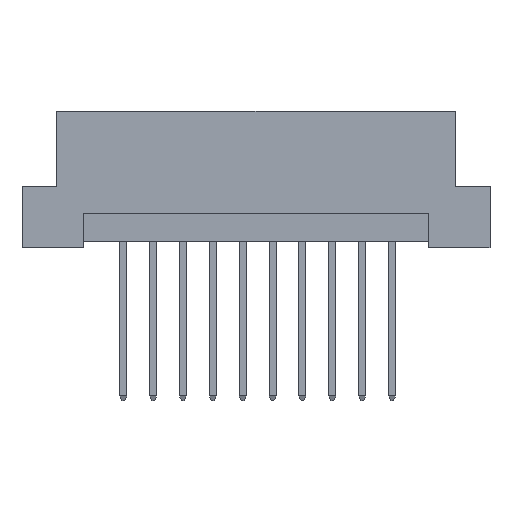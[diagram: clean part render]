
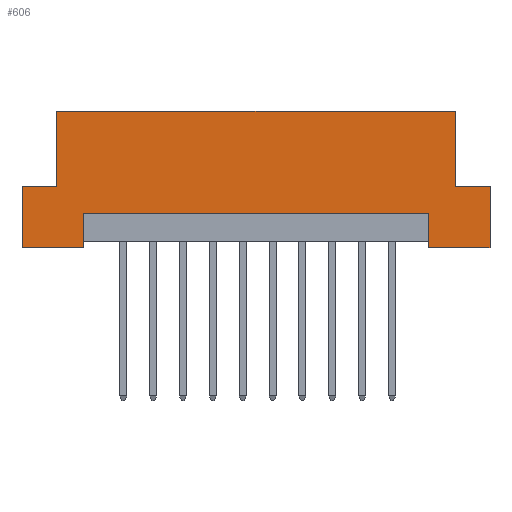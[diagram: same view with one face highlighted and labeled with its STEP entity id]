
A CAD part, front view. The second image highlights one B-rep face of the part: STEP entity #606.
In plain terms, the highlighted planar face has unit normal (0, -1, 0).
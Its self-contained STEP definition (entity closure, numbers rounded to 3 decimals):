
#6 = LINE ( 'NONE', #4077, #3075 ) ;
#26 = ORIENTED_EDGE ( 'NONE', *, *, #523, .F. ) ;
#90 = DIRECTION ( 'NONE',  ( -1., 0., 0. ) ) ;
#108 = DIRECTION ( 'NONE',  ( 0., 0., -1. ) ) ;
#235 = EDGE_CURVE ( 'NONE', #1384, #5717, #3863, .T. ) ;
#265 = VECTOR ( 'NONE', #2667, 1000. ) ;
#295 = CARTESIAN_POINT ( 'NONE',  ( -19.9, 0., 0. ) ) ;
#346 = EDGE_LOOP ( 'NONE', ( #26, #4946, #2214, #2042, #5143, #6350, #1174, #2642, #4425, #2897, #4144, #871 ) ) ;
#352 = LINE ( 'NONE', #419, #2236 ) ;
#419 = CARTESIAN_POINT ( 'NONE',  ( -19.9, 0., 0. ) ) ;
#425 = EDGE_CURVE ( 'NONE', #3949, #3758, #2984, .T. ) ;
#485 = DIRECTION ( 'NONE',  ( 0., 0., 1. ) ) ;
#523 = EDGE_CURVE ( 'NONE', #6024, #3803, #5255, .T. ) ;
#606 = ADVANCED_FACE ( 'NONE', ( #4904 ), #5379, .F. ) ;
#613 = LINE ( 'NONE', #5139, #684 ) ;
#618 = DIRECTION ( 'NONE',  ( 0., 0., -1. ) ) ;
#684 = VECTOR ( 'NONE', #108, 1000. ) ;
#708 = EDGE_CURVE ( 'NONE', #5141, #5516, #352, .T. ) ;
#871 = ORIENTED_EDGE ( 'NONE', *, *, #3981, .F. ) ;
#911 = DIRECTION ( 'NONE',  ( 1., 0., 0. ) ) ;
#1126 = CARTESIAN_POINT ( 'NONE',  ( 16.94, 0., 11.6 ) ) ;
#1157 = EDGE_CURVE ( 'NONE', #1899, #3949, #6, .T. ) ;
#1170 = VERTEX_POINT ( 'NONE', #6666 ) ;
#1174 = ORIENTED_EDGE ( 'NONE', *, *, #4488, .F. ) ;
#1384 = VERTEX_POINT ( 'NONE', #4988 ) ;
#1573 = CARTESIAN_POINT ( 'NONE',  ( -19.9, 0., 11.6 ) ) ;
#1659 = VECTOR ( 'NONE', #2355, 1000. ) ;
#1704 = CARTESIAN_POINT ( 'NONE',  ( -19.9, 0., 11.6 ) ) ;
#1819 = VECTOR ( 'NONE', #90, 1000. ) ;
#1820 = CARTESIAN_POINT ( 'NONE',  ( -14.69, 0., 0. ) ) ;
#1899 = VERTEX_POINT ( 'NONE', #6479 ) ;
#1977 = CARTESIAN_POINT ( 'NONE',  ( 19.9, 0., 0. ) ) ;
#2042 = ORIENTED_EDGE ( 'NONE', *, *, #425, .F. ) ;
#2144 = EDGE_CURVE ( 'NONE', #6024, #3431, #6234, .T. ) ;
#2214 = ORIENTED_EDGE ( 'NONE', *, *, #3253, .F. ) ;
#2236 = VECTOR ( 'NONE', #6577, 1000. ) ;
#2355 = DIRECTION ( 'NONE',  ( 0., 0., 1. ) ) ;
#2457 = DIRECTION ( 'NONE',  ( 1., 0., 0. ) ) ;
#2591 = EDGE_CURVE ( 'NONE', #1170, #1384, #3984, .T. ) ;
#2642 = ORIENTED_EDGE ( 'NONE', *, *, #235, .F. ) ;
#2661 = LINE ( 'NONE', #5304, #1659 ) ;
#2667 = DIRECTION ( 'NONE',  ( 1., 0., 0. ) ) ;
#2709 = VECTOR ( 'NONE', #6482, 1000. ) ;
#2897 = ORIENTED_EDGE ( 'NONE', *, *, #6393, .F. ) ;
#2984 = LINE ( 'NONE', #1977, #6591 ) ;
#3038 = VECTOR ( 'NONE', #2457, 1000. ) ;
#3053 = VECTOR ( 'NONE', #485, 1000. ) ;
#3075 = VECTOR ( 'NONE', #911, 1000. ) ;
#3253 = EDGE_CURVE ( 'NONE', #3758, #3431, #4838, .T. ) ;
#3431 = VERTEX_POINT ( 'NONE', #5046 ) ;
#3484 = CARTESIAN_POINT ( 'NONE',  ( -19.9, 0., 5.2 ) ) ;
#3758 = VERTEX_POINT ( 'NONE', #4424 ) ;
#3803 = VERTEX_POINT ( 'NONE', #5610 ) ;
#3826 = DIRECTION ( 'NONE',  ( 0., 0., 1. ) ) ;
#3863 = LINE ( 'NONE', #5459, #5161 ) ;
#3875 = EDGE_CURVE ( 'NONE', #1899, #4615, #6090, .T. ) ;
#3892 = DIRECTION ( 'NONE',  ( 0., 0., 1. ) ) ;
#3949 = VERTEX_POINT ( 'NONE', #5785 ) ;
#3981 = EDGE_CURVE ( 'NONE', #3803, #5141, #613, .T. ) ;
#3984 = LINE ( 'NONE', #3484, #3038 ) ;
#3985 = CARTESIAN_POINT ( 'NONE',  ( 16.94, 0., 5.2 ) ) ;
#4077 = CARTESIAN_POINT ( 'NONE',  ( 19.9, 0., 5.2 ) ) ;
#4144 = ORIENTED_EDGE ( 'NONE', *, *, #708, .F. ) ;
#4300 = CARTESIAN_POINT ( 'NONE',  ( 14.69, 0., 2.9 ) ) ;
#4424 = CARTESIAN_POINT ( 'NONE',  ( 19.9, 0., 0. ) ) ;
#4425 = ORIENTED_EDGE ( 'NONE', *, *, #2591, .F. ) ;
#4475 = CARTESIAN_POINT ( 'NONE',  ( -16.94, 0., 11.6 ) ) ;
#4488 = EDGE_CURVE ( 'NONE', #5717, #4615, #5658, .T. ) ;
#4615 = VERTEX_POINT ( 'NONE', #1126 ) ;
#4640 = CARTESIAN_POINT ( 'NONE',  ( 14.69, 0., 2.9 ) ) ;
#4762 = CARTESIAN_POINT ( 'NONE',  ( 14.69, 0., 0.5 ) ) ;
#4838 = LINE ( 'NONE', #4977, #2709 ) ;
#4904 = FACE_OUTER_BOUND ( 'NONE', #346, .T. ) ;
#4946 = ORIENTED_EDGE ( 'NONE', *, *, #2144, .T. ) ;
#4977 = CARTESIAN_POINT ( 'NONE',  ( -19.9, 0., 0. ) ) ;
#4988 = CARTESIAN_POINT ( 'NONE',  ( -16.94, 0., 5.2 ) ) ;
#5046 = CARTESIAN_POINT ( 'NONE',  ( 14.69, 0., 0. ) ) ;
#5050 = DIRECTION ( 'NONE',  ( 0., 0., -1. ) ) ;
#5139 = CARTESIAN_POINT ( 'NONE',  ( -14.69, 0., 0.5 ) ) ;
#5141 = VERTEX_POINT ( 'NONE', #1820 ) ;
#5143 = ORIENTED_EDGE ( 'NONE', *, *, #1157, .F. ) ;
#5161 = VECTOR ( 'NONE', #3892, 1000. ) ;
#5255 = LINE ( 'NONE', #4640, #1819 ) ;
#5304 = CARTESIAN_POINT ( 'NONE',  ( -19.9, 0., 0. ) ) ;
#5379 = PLANE ( 'NONE',  #6139 ) ;
#5459 = CARTESIAN_POINT ( 'NONE',  ( -16.94, 0., 5.2 ) ) ;
#5516 = VERTEX_POINT ( 'NONE', #295 ) ;
#5610 = CARTESIAN_POINT ( 'NONE',  ( -14.69, 0., 2.9 ) ) ;
#5658 = LINE ( 'NONE', #1573, #265 ) ;
#5717 = VERTEX_POINT ( 'NONE', #4475 ) ;
#5785 = CARTESIAN_POINT ( 'NONE',  ( 19.9, 0., 5.2 ) ) ;
#5804 = VECTOR ( 'NONE', #618, 1000. ) ;
#5858 = DIRECTION ( 'NONE',  ( 0., 1., 0. ) ) ;
#6024 = VERTEX_POINT ( 'NONE', #4300 ) ;
#6090 = LINE ( 'NONE', #3985, #3053 ) ;
#6139 = AXIS2_PLACEMENT_3D ( 'NONE', #1704, #5858, #3826 ) ;
#6234 = LINE ( 'NONE', #4762, #5804 ) ;
#6350 = ORIENTED_EDGE ( 'NONE', *, *, #3875, .T. ) ;
#6393 = EDGE_CURVE ( 'NONE', #5516, #1170, #2661, .T. ) ;
#6479 = CARTESIAN_POINT ( 'NONE',  ( 16.94, 0., 5.2 ) ) ;
#6482 = DIRECTION ( 'NONE',  ( -1., 0., 0. ) ) ;
#6577 = DIRECTION ( 'NONE',  ( -1., 0., 0. ) ) ;
#6591 = VECTOR ( 'NONE', #5050, 1000. ) ;
#6666 = CARTESIAN_POINT ( 'NONE',  ( -19.9, 0., 5.2 ) ) ;
